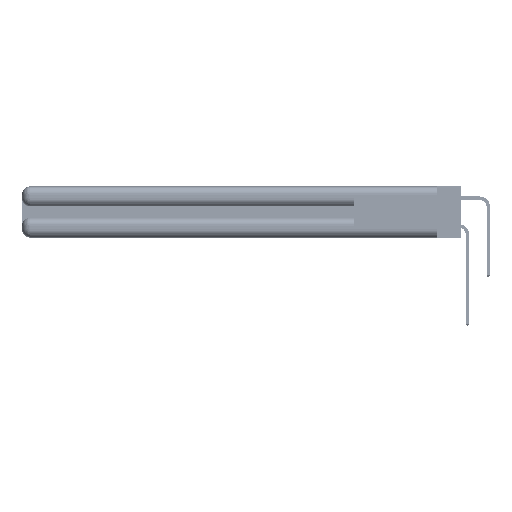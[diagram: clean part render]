
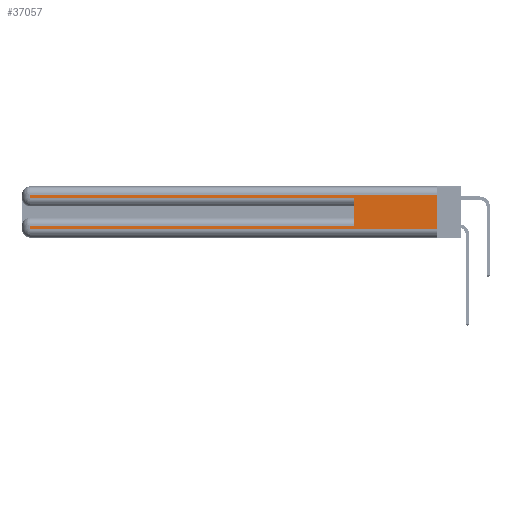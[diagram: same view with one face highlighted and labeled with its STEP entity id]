
A CAD part, left-side view. The second image highlights one B-rep face of the part: STEP entity #37057.
In plain terms, the highlighted planar face has unit normal (-1, 0, 0).
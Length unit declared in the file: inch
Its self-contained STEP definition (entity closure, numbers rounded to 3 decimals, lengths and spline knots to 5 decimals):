
#66 = ORIENTED_EDGE ( 'NONE', *, *, #16625, .T. ) ;
#257 = DIRECTION ( 'NONE',  ( 0., -1., 0. ) ) ;
#289 = LINE ( 'NONE', #10327, #11060 ) ;
#3540 = CARTESIAN_POINT ( 'NONE',  ( 0., 0., 0.31 ) ) ;
#5824 = ORIENTED_EDGE ( 'NONE', *, *, #54873, .T. ) ;
#5998 = CARTESIAN_POINT ( 'NONE',  ( 0., 0.6, 0.085 ) ) ;
#6499 = ORIENTED_EDGE ( 'NONE', *, *, #44251, .T. ) ;
#7621 = EDGE_CURVE ( 'NONE', #58229, #30503, #45038, .T. ) ;
#7679 = PLANE ( 'NONE',  #47670 ) ;
#8354 = CARTESIAN_POINT ( 'NONE',  ( 0., 2.94, 0.085 ) ) ;
#9172 = VERTEX_POINT ( 'NONE', #25498 ) ;
#10327 = CARTESIAN_POINT ( 'NONE',  ( 0., 0., 0.06 ) ) ;
#10875 = CARTESIAN_POINT ( 'NONE',  ( 0., 0., 0.085 ) ) ;
#11060 = VECTOR ( 'NONE', #15235, 39.37008 ) ;
#11336 = CARTESIAN_POINT ( 'NONE',  ( 0., 2.94, 0.37 ) ) ;
#12079 = VECTOR ( 'NONE', #43466, 39.37008 ) ;
#12873 = CARTESIAN_POINT ( 'NONE',  ( 0., 2.94, 0.37 ) ) ;
#12983 = EDGE_CURVE ( 'NONE', #21445, #50712, #289, .T. ) ;
#13015 = ORIENTED_EDGE ( 'NONE', *, *, #26620, .T. ) ;
#15235 = DIRECTION ( 'NONE',  ( 0., -1., 0. ) ) ;
#15701 = VERTEX_POINT ( 'NONE', #57937 ) ;
#16625 = EDGE_CURVE ( 'NONE', #15701, #30503, #53783, .T. ) ;
#16838 = DIRECTION ( 'NONE',  ( 1., 0., 0. ) ) ;
#17034 = DIRECTION ( 'NONE',  ( 0., 0., -1. ) ) ;
#17307 = CARTESIAN_POINT ( 'NONE',  ( 0., 2.94, 0.06 ) ) ;
#17571 = DIRECTION ( 'NONE',  ( 0., 0., -1. ) ) ;
#18677 = VECTOR ( 'NONE', #257, 39.37008 ) ;
#18683 = DIRECTION ( 'NONE',  ( 0., 0., 1. ) ) ;
#19075 = DIRECTION ( 'NONE',  ( 0., 0., -1. ) ) ;
#20654 = LINE ( 'NONE', #3540, #31430 ) ;
#20976 = VECTOR ( 'NONE', #19075, 39.37008 ) ;
#21445 = VERTEX_POINT ( 'NONE', #17307 ) ;
#22423 = LINE ( 'NONE', #23658, #20976 ) ;
#22897 = LINE ( 'NONE', #11336, #12079 ) ;
#23658 = CARTESIAN_POINT ( 'NONE',  ( 0., 0., 0.37 ) ) ;
#24421 = FACE_OUTER_BOUND ( 'NONE', #29917, .T. ) ;
#25498 = CARTESIAN_POINT ( 'NONE',  ( 0., 0., 0.31 ) ) ;
#25727 = CARTESIAN_POINT ( 'NONE',  ( 0., 0.6, 0.285 ) ) ;
#26620 = EDGE_CURVE ( 'NONE', #9172, #30915, #20654, .T. ) ;
#27823 = CARTESIAN_POINT ( 'NONE',  ( 0., 0., 0.285 ) ) ;
#29325 = EDGE_CURVE ( 'NONE', #9172, #50712, #22423, .T. ) ;
#29753 = CARTESIAN_POINT ( 'NONE',  ( 0., 0., 0.06 ) ) ;
#29917 = EDGE_LOOP ( 'NONE', ( #33156, #13015, #6499, #66, #36790, #41078, #5824, #33199 ) ) ;
#30503 = VERTEX_POINT ( 'NONE', #25727 ) ;
#30915 = VERTEX_POINT ( 'NONE', #37733 ) ;
#31430 = VECTOR ( 'NONE', #35715, 39.37008 ) ;
#33156 = ORIENTED_EDGE ( 'NONE', *, *, #29325, .F. ) ;
#33199 = ORIENTED_EDGE ( 'NONE', *, *, #12983, .T. ) ;
#33834 = DIRECTION ( 'NONE',  ( 0., 1., 0. ) ) ;
#34216 = LINE ( 'NONE', #12873, #58576 ) ;
#35715 = DIRECTION ( 'NONE',  ( 0., 1., 0. ) ) ;
#36790 = ORIENTED_EDGE ( 'NONE', *, *, #7621, .F. ) ;
#37057 = ADVANCED_FACE ( 'NONE', ( #24421 ), #7679, .F. ) ;
#37733 = CARTESIAN_POINT ( 'NONE',  ( 0., 2.94, 0.31 ) ) ;
#41078 = ORIENTED_EDGE ( 'NONE', *, *, #57556, .T. ) ;
#42834 = LINE ( 'NONE', #10875, #53630 ) ;
#43466 = DIRECTION ( 'NONE',  ( 0., 0., -1. ) ) ;
#43928 = VERTEX_POINT ( 'NONE', #8354 ) ;
#44071 = CARTESIAN_POINT ( 'NONE',  ( 0., 0., 0.37 ) ) ;
#44251 = EDGE_CURVE ( 'NONE', #30915, #15701, #22897, .T. ) ;
#45038 = LINE ( 'NONE', #46133, #57184 ) ;
#46133 = CARTESIAN_POINT ( 'NONE',  ( 0., 0.6, 0.145 ) ) ;
#47670 = AXIS2_PLACEMENT_3D ( 'NONE', #44071, #16838, #17034 ) ;
#50712 = VERTEX_POINT ( 'NONE', #29753 ) ;
#53630 = VECTOR ( 'NONE', #33834, 39.37008 ) ;
#53783 = LINE ( 'NONE', #27823, #18677 ) ;
#54873 = EDGE_CURVE ( 'NONE', #43928, #21445, #34216, .T. ) ;
#57184 = VECTOR ( 'NONE', #18683, 39.37008 ) ;
#57556 = EDGE_CURVE ( 'NONE', #58229, #43928, #42834, .T. ) ;
#57937 = CARTESIAN_POINT ( 'NONE',  ( 0., 2.94, 0.285 ) ) ;
#58229 = VERTEX_POINT ( 'NONE', #5998 ) ;
#58576 = VECTOR ( 'NONE', #17571, 39.37008 ) ;
